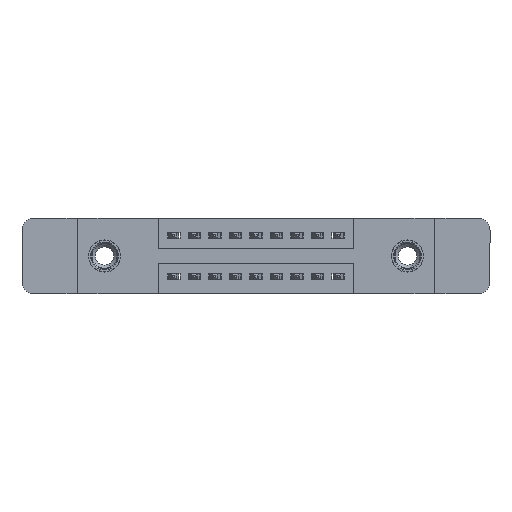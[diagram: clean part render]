
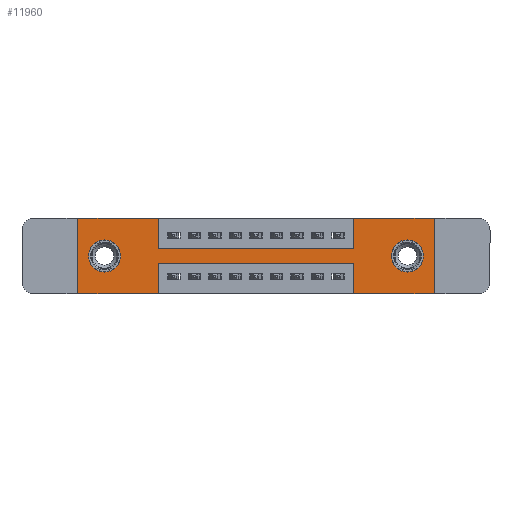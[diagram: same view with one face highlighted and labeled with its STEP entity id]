
A CAD part, front view. The second image highlights one B-rep face of the part: STEP entity #11960.
In plain terms, the highlighted planar face has unit normal (0, -1, 0).
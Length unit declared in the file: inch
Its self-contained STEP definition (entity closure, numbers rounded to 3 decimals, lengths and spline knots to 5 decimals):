
#156 = ORIENTED_EDGE ( 'NONE', *, *, #16183, .F. ) ;
#173 = EDGE_CURVE ( 'NONE', #3286, #7436, #7758, .T. ) ;
#278 = VERTEX_POINT ( 'NONE', #5625 ) ;
#279 = EDGE_LOOP ( 'NONE', ( #7642, #11031 ) ) ;
#347 = ORIENTED_EDGE ( 'NONE', *, *, #173, .F. ) ;
#573 = CARTESIAN_POINT ( 'NONE',  ( 1.3425, 0., -0.37 ) ) ;
#782 = CARTESIAN_POINT ( 'NONE',  ( 1.605, 0., -0.185 ) ) ;
#996 = CARTESIAN_POINT ( 'NONE',  ( 1.735, 0., -0.37 ) ) ;
#1019 = DIRECTION ( 'NONE',  ( 1., 0., 0. ) ) ;
#1166 = ORIENTED_EDGE ( 'NONE', *, *, #2787, .T. ) ;
#1391 = CARTESIAN_POINT ( 'NONE',  ( 0., 0., 0. ) ) ;
#1440 = CARTESIAN_POINT ( 'NONE',  ( 1.605, 0., -0.107 ) ) ;
#1571 = ORIENTED_EDGE ( 'NONE', *, *, #8181, .F. ) ;
#1810 = CARTESIAN_POINT ( 'NONE',  ( 1.735, 0., 0. ) ) ;
#2051 = CARTESIAN_POINT ( 'NONE',  ( 1.605, 0., -0.263 ) ) ;
#2149 = ORIENTED_EDGE ( 'NONE', *, *, #16502, .F. ) ;
#2184 = VERTEX_POINT ( 'NONE', #5019 ) ;
#2269 = DIRECTION ( 'NONE',  ( 0., 1., 0. ) ) ;
#2369 = CIRCLE ( 'NONE', #7983, 0.078 ) ;
#2515 = PLANE ( 'NONE',  #3396 ) ;
#2572 = CARTESIAN_POINT ( 'NONE',  ( 0.3925, 0., -0.15 ) ) ;
#2713 = VERTEX_POINT ( 'NONE', #1440 ) ;
#2787 = EDGE_CURVE ( 'NONE', #2713, #10310, #12497, .T. ) ;
#2904 = FACE_BOUND ( 'NONE', #11375, .T. ) ;
#3000 = VECTOR ( 'NONE', #14017, 39.37008 ) ;
#3054 = CARTESIAN_POINT ( 'NONE',  ( 1.3425, 0., 0. ) ) ;
#3102 = CARTESIAN_POINT ( 'NONE',  ( 0., 0., 0. ) ) ;
#3200 = VECTOR ( 'NONE', #1019, 39.37008 ) ;
#3286 = VERTEX_POINT ( 'NONE', #9088 ) ;
#3320 = ORIENTED_EDGE ( 'NONE', *, *, #5366, .F. ) ;
#3377 = LINE ( 'NONE', #1810, #8235 ) ;
#3396 = AXIS2_PLACEMENT_3D ( 'NONE', #14137, #6428, #7723 ) ;
#3477 = VECTOR ( 'NONE', #4507, 39.37008 ) ;
#3777 = EDGE_CURVE ( 'NONE', #278, #12383, #2369, .T. ) ;
#3806 = LINE ( 'NONE', #11326, #3200 ) ;
#4036 = LINE ( 'NONE', #3102, #15344 ) ;
#4321 = DIRECTION ( 'NONE',  ( 0., 0., -1. ) ) ;
#4507 = DIRECTION ( 'NONE',  ( 0., 0., -1. ) ) ;
#5019 = CARTESIAN_POINT ( 'NONE',  ( 0.3925, 0., -0.37 ) ) ;
#5094 = DIRECTION ( 'NONE',  ( 1., 0., 0. ) ) ;
#5164 = DIRECTION ( 'NONE',  ( -1., 0., 0. ) ) ;
#5176 = LINE ( 'NONE', #573, #12392 ) ;
#5366 = EDGE_CURVE ( 'NONE', #11550, #10859, #5176, .T. ) ;
#5379 = CARTESIAN_POINT ( 'NONE',  ( 1.3425, 0., -0.15 ) ) ;
#5439 = DIRECTION ( 'NONE',  ( 0., 0., -1. ) ) ;
#5625 = CARTESIAN_POINT ( 'NONE',  ( 0.13, 0., -0.107 ) ) ;
#5731 = LINE ( 'NONE', #10740, #11360 ) ;
#6428 = DIRECTION ( 'NONE',  ( 0., -1., 0. ) ) ;
#6911 = CARTESIAN_POINT ( 'NONE',  ( 0., 0., -0.37 ) ) ;
#6913 = CARTESIAN_POINT ( 'NONE',  ( 0.13, 0., -0.185 ) ) ;
#7118 = VERTEX_POINT ( 'NONE', #3054 ) ;
#7413 = CARTESIAN_POINT ( 'NONE',  ( 1.3425, 0., -0.37 ) ) ;
#7436 = VERTEX_POINT ( 'NONE', #5379 ) ;
#7443 = CIRCLE ( 'NONE', #9473, 0.078 ) ;
#7640 = EDGE_CURVE ( 'NONE', #10859, #12461, #11567, .T. ) ;
#7642 = ORIENTED_EDGE ( 'NONE', *, *, #3777, .T. ) ;
#7723 = DIRECTION ( 'NONE',  ( 0., 0., -1. ) ) ;
#7735 = VERTEX_POINT ( 'NONE', #996 ) ;
#7758 = LINE ( 'NONE', #2572, #15809 ) ;
#7983 = AXIS2_PLACEMENT_3D ( 'NONE', #6913, #15874, #9486 ) ;
#8017 = DIRECTION ( 'NONE',  ( 0., 0., -1. ) ) ;
#8181 = EDGE_CURVE ( 'NONE', #16184, #9630, #13375, .T. ) ;
#8235 = VECTOR ( 'NONE', #4321, 39.37008 ) ;
#8313 = VECTOR ( 'NONE', #15923, 39.37008 ) ;
#8407 = CARTESIAN_POINT ( 'NONE',  ( 0.3925, 0., -0.37 ) ) ;
#8597 = ORIENTED_EDGE ( 'NONE', *, *, #12585, .F. ) ;
#8738 = VECTOR ( 'NONE', #5439, 39.37008 ) ;
#8933 = LINE ( 'NONE', #6911, #8313 ) ;
#9030 = CARTESIAN_POINT ( 'NONE',  ( 0.3925, 0., -0.22 ) ) ;
#9051 = VERTEX_POINT ( 'NONE', #13719 ) ;
#9088 = CARTESIAN_POINT ( 'NONE',  ( 0.3925, 0., -0.15 ) ) ;
#9097 = ORIENTED_EDGE ( 'NONE', *, *, #14150, .F. ) ;
#9108 = CARTESIAN_POINT ( 'NONE',  ( 0., 0., 0. ) ) ;
#9209 = CARTESIAN_POINT ( 'NONE',  ( 0.3925, 0., -0.22 ) ) ;
#9473 = AXIS2_PLACEMENT_3D ( 'NONE', #15883, #9553, #13398 ) ;
#9486 = DIRECTION ( 'NONE',  ( 0., 0., 1. ) ) ;
#9553 = DIRECTION ( 'NONE',  ( 0., 1., 0. ) ) ;
#9630 = VERTEX_POINT ( 'NONE', #12931 ) ;
#9967 = CARTESIAN_POINT ( 'NONE',  ( 1.735, 0., 0. ) ) ;
#10003 = CIRCLE ( 'NONE', #10125, 0.078 ) ;
#10125 = AXIS2_PLACEMENT_3D ( 'NONE', #12045, #15731, #8017 ) ;
#10310 = VERTEX_POINT ( 'NONE', #2051 ) ;
#10331 = CARTESIAN_POINT ( 'NONE',  ( 1.3425, 0., 0. ) ) ;
#10508 = EDGE_CURVE ( 'NONE', #7118, #11403, #3806, .T. ) ;
#10555 = EDGE_CURVE ( 'NONE', #12383, #278, #7443, .T. ) ;
#10573 = FACE_OUTER_BOUND ( 'NONE', #13767, .T. ) ;
#10740 = CARTESIAN_POINT ( 'NONE',  ( 0., 0., -0.37 ) ) ;
#10859 = VERTEX_POINT ( 'NONE', #13604 ) ;
#11031 = ORIENTED_EDGE ( 'NONE', *, *, #10555, .T. ) ;
#11117 = ORIENTED_EDGE ( 'NONE', *, *, #7640, .F. ) ;
#11163 = VECTOR ( 'NONE', #5164, 39.37008 ) ;
#11326 = CARTESIAN_POINT ( 'NONE',  ( 0., 0., 0. ) ) ;
#11360 = VECTOR ( 'NONE', #12115, 39.37008 ) ;
#11375 = EDGE_LOOP ( 'NONE', ( #1166, #13149 ) ) ;
#11403 = VERTEX_POINT ( 'NONE', #9967 ) ;
#11434 = EDGE_CURVE ( 'NONE', #10310, #2713, #10003, .T. ) ;
#11456 = ORIENTED_EDGE ( 'NONE', *, *, #10508, .F. ) ;
#11550 = VERTEX_POINT ( 'NONE', #7413 ) ;
#11567 = LINE ( 'NONE', #9030, #11163 ) ;
#11926 = AXIS2_PLACEMENT_3D ( 'NONE', #782, #2269, #12980 ) ;
#11960 = ADVANCED_FACE ( 'NONE', ( #2904, #12163, #10573 ), #2515, .T. ) ;
#12045 = CARTESIAN_POINT ( 'NONE',  ( 1.605, 0., -0.185 ) ) ;
#12115 = DIRECTION ( 'NONE',  ( -1., 0., 0. ) ) ;
#12163 = FACE_BOUND ( 'NONE', #279, .T. ) ;
#12338 = LINE ( 'NONE', #8407, #3477 ) ;
#12383 = VERTEX_POINT ( 'NONE', #15232 ) ;
#12392 = VECTOR ( 'NONE', #16156, 39.37008 ) ;
#12461 = VERTEX_POINT ( 'NONE', #9209 ) ;
#12497 = CIRCLE ( 'NONE', #11926, 0.078 ) ;
#12585 = EDGE_CURVE ( 'NONE', #9630, #3286, #14583, .T. ) ;
#12931 = CARTESIAN_POINT ( 'NONE',  ( 0.3925, 0., 0. ) ) ;
#12980 = DIRECTION ( 'NONE',  ( 0., 0., -1. ) ) ;
#13149 = ORIENTED_EDGE ( 'NONE', *, *, #11434, .T. ) ;
#13201 = CARTESIAN_POINT ( 'NONE',  ( 0.3925, 0., 0. ) ) ;
#13207 = EDGE_CURVE ( 'NONE', #7735, #11550, #5731, .T. ) ;
#13260 = ORIENTED_EDGE ( 'NONE', *, *, #15162, .F. ) ;
#13375 = LINE ( 'NONE', #1391, #13753 ) ;
#13398 = DIRECTION ( 'NONE',  ( 0., 0., 1. ) ) ;
#13561 = DIRECTION ( 'NONE',  ( 0., 0., 1. ) ) ;
#13604 = CARTESIAN_POINT ( 'NONE',  ( 1.3425, 0., -0.22 ) ) ;
#13624 = EDGE_CURVE ( 'NONE', #12461, #2184, #12338, .T. ) ;
#13719 = CARTESIAN_POINT ( 'NONE',  ( 0., 0., -0.37 ) ) ;
#13753 = VECTOR ( 'NONE', #5094, 39.37008 ) ;
#13767 = EDGE_LOOP ( 'NONE', ( #14942, #11117, #3320, #14303, #2149, #11456, #156, #347, #8597, #1571, #13260, #9097 ) ) ;
#14017 = DIRECTION ( 'NONE',  ( 0., 0., 1. ) ) ;
#14137 = CARTESIAN_POINT ( 'NONE',  ( 0., 0., -0.37 ) ) ;
#14150 = EDGE_CURVE ( 'NONE', #2184, #9051, #8933, .T. ) ;
#14303 = ORIENTED_EDGE ( 'NONE', *, *, #13207, .F. ) ;
#14583 = LINE ( 'NONE', #13201, #8738 ) ;
#14942 = ORIENTED_EDGE ( 'NONE', *, *, #13624, .F. ) ;
#15162 = EDGE_CURVE ( 'NONE', #9051, #16184, #4036, .T. ) ;
#15232 = CARTESIAN_POINT ( 'NONE',  ( 0.13, 0., -0.263 ) ) ;
#15344 = VECTOR ( 'NONE', #13561, 39.37008 ) ;
#15731 = DIRECTION ( 'NONE',  ( 0., 1., 0. ) ) ;
#15809 = VECTOR ( 'NONE', #16550, 39.37008 ) ;
#15874 = DIRECTION ( 'NONE',  ( 0., 1., 0. ) ) ;
#15883 = CARTESIAN_POINT ( 'NONE',  ( 0.13, 0., -0.185 ) ) ;
#15923 = DIRECTION ( 'NONE',  ( -1., 0., 0. ) ) ;
#16156 = DIRECTION ( 'NONE',  ( 0., 0., 1. ) ) ;
#16183 = EDGE_CURVE ( 'NONE', #7436, #7118, #16490, .T. ) ;
#16184 = VERTEX_POINT ( 'NONE', #9108 ) ;
#16490 = LINE ( 'NONE', #10331, #3000 ) ;
#16502 = EDGE_CURVE ( 'NONE', #11403, #7735, #3377, .T. ) ;
#16550 = DIRECTION ( 'NONE',  ( 1., 0., 0. ) ) ;
